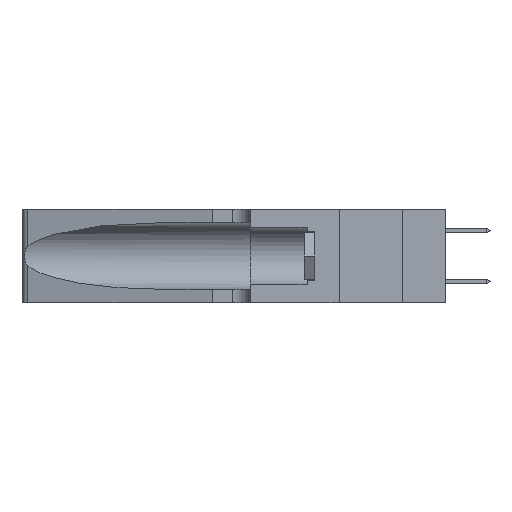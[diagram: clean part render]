
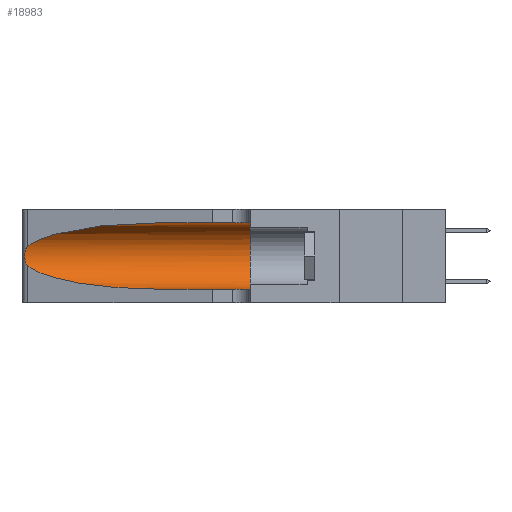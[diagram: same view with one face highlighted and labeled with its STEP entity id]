
A CAD part, left-side view. The second image highlights one B-rep face of the part: STEP entity #18983.
In plain terms, the highlighted cylindrical face has radius 3.308 mm (diameter 6.617 mm), a partial arc.
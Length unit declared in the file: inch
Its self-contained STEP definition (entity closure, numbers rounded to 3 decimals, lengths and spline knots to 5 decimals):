
#10 = FACE_OUTER_BOUND ( 'NONE', #20037, .T. ) ;
#202 = LINE ( 'NONE', #22801, #10548 ) ;
#737 = B_SPLINE_CURVE_WITH_KNOTS ( 'NONE', 3,
 ( #7011, #8962, #22383, #10937, #24310, #12885, #1257, #14824, #3184, #16738, #5118, #18635, #7104, #20547 ),
 .UNSPECIFIED., .F., .F.,
 ( 4, 2, 2, 2, 2, 2, 4 ),
 ( 0., 0.00027, 0.00053, 0.00107, 0.0016, 0.00187, 0.00214 ),
 .UNSPECIFIED. ) ;
#758 = VERTEX_POINT ( 'NONE', #13399 ) ;
#1257 = CARTESIAN_POINT ( 'NONE',  ( 0.26075, 1.23896, 0.19203 ) ) ;
#1822 = AXIS2_PLACEMENT_3D ( 'NONE', #2284, #15841, #4201 ) ;
#2284 = CARTESIAN_POINT ( 'NONE',  ( 0.1305, 0.35, 0.185 ) ) ;
#2355 = CARTESIAN_POINT ( 'NONE',  ( 0.18966, 0.96281, 0.05475 ) ) ;
#3184 = CARTESIAN_POINT ( 'NONE',  ( 0.26017, 1.23833, 0.17102 ) ) ;
#3307 = CARTESIAN_POINT ( 'NONE',  ( 0.1305, 0.72297, 0.31525 ) ) ;
#3493 = DIRECTION ( 'NONE',  ( 0., -1., 0. ) ) ;
#3822 = EDGE_CURVE ( 'NONE', #12488, #758, #737, .T. ) ;
#4157 = CARTESIAN_POINT ( 'NONE',  ( 0.25487, 1.22718, 0.22369 ) ) ;
#4201 = DIRECTION ( 'NONE',  ( 0., 0., 1. ) ) ;
#4568 = CYLINDRICAL_SURFACE ( 'NONE', #11282, 0.13025 ) ;
#5118 = CARTESIAN_POINT ( 'NONE',  ( 0.25789, 1.23486, 0.15765 ) ) ;
#5637 = DIRECTION ( 'NONE',  ( 0., -1., 0. ) ) ;
#5681 =( BOUNDED_CURVE ( )  B_SPLINE_CURVE ( 3, ( #12040, #13962, #2355, #15912 ),
 .UNSPECIFIED., .F., .F. ) 
 B_SPLINE_CURVE_WITH_KNOTS ( ( 4, 4 ),
 ( 3.44316, 4.71239 ),
 .UNSPECIFIED. ) 
 CURVE ( )  GEOMETRIC_REPRESENTATION_ITEM ( )  RATIONAL_B_SPLINE_CURVE ( ( 1., 0.87, 0.87, 1. ) ) 
 REPRESENTATION_ITEM ( '' )  );
#6801 = CARTESIAN_POINT ( 'NONE',  ( 0.1305, 0.72297, 0.05475 ) ) ;
#7011 = CARTESIAN_POINT ( 'NONE',  ( 0.25487, 1.22718, 0.22369 ) ) ;
#7104 = CARTESIAN_POINT ( 'NONE',  ( 0.25555, 1.22993, 0.14849 ) ) ;
#7156 = EDGE_CURVE ( 'NONE', #19584, #22813, #21351, .T. ) ;
#7575 = CARTESIAN_POINT ( 'NONE',  ( 0.1305, 0.35, 0.31525 ) ) ;
#7622 = EDGE_CURVE ( 'NONE', #23781, #19584, #202, .T. ) ;
#7841 = CARTESIAN_POINT ( 'NONE',  ( 0.25487, 1.22718, 0.22369 ) ) ;
#8809 = ORIENTED_EDGE ( 'NONE', *, *, #7622, .F. ) ;
#8962 = CARTESIAN_POINT ( 'NONE',  ( 0.25555, 1.22994, 0.2215 ) ) ;
#10548 = VECTOR ( 'NONE', #18960, 39.37008 ) ;
#10937 = CARTESIAN_POINT ( 'NONE',  ( 0.25787, 1.23484, 0.2124 ) ) ;
#11282 = AXIS2_PLACEMENT_3D ( 'NONE', #22989, #5637, #13385 ) ;
#11324 = ORIENTED_EDGE ( 'NONE', *, *, #7156, .F. ) ;
#11931 = CARTESIAN_POINT ( 'NONE',  ( 0.1305, 0.72297, 0.31525 ) ) ;
#12040 = CARTESIAN_POINT ( 'NONE',  ( 0.25487, 1.22718, 0.14631 ) ) ;
#12488 = VERTEX_POINT ( 'NONE', #7841 ) ;
#12885 = CARTESIAN_POINT ( 'NONE',  ( 0.26018, 1.23835, 0.19895 ) ) ;
#13385 = DIRECTION ( 'NONE',  ( 0., 0., -1. ) ) ;
#13399 = CARTESIAN_POINT ( 'NONE',  ( 0.25487, 1.22718, 0.14631 ) ) ;
#13962 = CARTESIAN_POINT ( 'NONE',  ( 0.2373, 1.15595, 0.08982 ) ) ;
#14727 = ORIENTED_EDGE ( 'NONE', *, *, #19130, .T. ) ;
#14824 = CARTESIAN_POINT ( 'NONE',  ( 0.26075, 1.23896, 0.178 ) ) ;
#14996 = ORIENTED_EDGE ( 'NONE', *, *, #16988, .T. ) ;
#15588 = CARTESIAN_POINT ( 'NONE',  ( 0.1305, 0.35, 0.05475 ) ) ;
#15790 = CARTESIAN_POINT ( 'NONE',  ( 0.2373, 1.15595, 0.28018 ) ) ;
#15841 = DIRECTION ( 'NONE',  ( 0., 1., 0. ) ) ;
#15912 = CARTESIAN_POINT ( 'NONE',  ( 0.1305, 0.72297, 0.05475 ) ) ;
#16291 = ORIENTED_EDGE ( 'NONE', *, *, #3822, .T. ) ;
#16738 = CARTESIAN_POINT ( 'NONE',  ( 0.25856, 1.23593, 0.16098 ) ) ;
#16988 = EDGE_CURVE ( 'NONE', #19942, #22813, #24857, .T. ) ;
#18635 = CARTESIAN_POINT ( 'NONE',  ( 0.25639, 1.23186, 0.15144 ) ) ;
#18940 = CARTESIAN_POINT ( 'NONE',  ( 0.1305, 1.61858, 0.05475 ) ) ;
#18960 = DIRECTION ( 'NONE',  ( 0., -1., 0. ) ) ;
#18983 = ADVANCED_FACE ( 'NONE', ( #10 ), #4568, .F. ) ;
#19130 = EDGE_CURVE ( 'NONE', #758, #19942, #5681, .T. ) ;
#19514 = CARTESIAN_POINT ( 'NONE',  ( 0.18966, 0.96281, 0.31525 ) ) ;
#19584 = VERTEX_POINT ( 'NONE', #7575 ) ;
#19713 = EDGE_CURVE ( 'NONE', #23781, #12488, #21723, .T. ) ;
#19765 = VECTOR ( 'NONE', #3493, 39.37008 ) ;
#19942 = VERTEX_POINT ( 'NONE', #6801 ) ;
#20037 = EDGE_LOOP ( 'NONE', ( #20341, #16291, #14727, #14996, #11324, #8809 ) ) ;
#20341 = ORIENTED_EDGE ( 'NONE', *, *, #19713, .T. ) ;
#20547 = CARTESIAN_POINT ( 'NONE',  ( 0.25487, 1.22718, 0.14631 ) ) ;
#21351 = CIRCLE ( 'NONE', #1822, 0.13025 ) ;
#21723 =( BOUNDED_CURVE ( )  B_SPLINE_CURVE ( 3, ( #11931, #19514, #15790, #4157 ),
 .UNSPECIFIED., .F., .T. ) 
 B_SPLINE_CURVE_WITH_KNOTS ( ( 4, 4 ),
 ( 1.5708, 2.84003 ),
 .UNSPECIFIED. ) 
 CURVE ( )  GEOMETRIC_REPRESENTATION_ITEM ( )  RATIONAL_B_SPLINE_CURVE ( ( 1., 0.87, 0.87, 1. ) ) 
 REPRESENTATION_ITEM ( '' )  );
#22383 = CARTESIAN_POINT ( 'NONE',  ( 0.25639, 1.23184, 0.21858 ) ) ;
#22801 = CARTESIAN_POINT ( 'NONE',  ( 0.1305, 1.61858, 0.31525 ) ) ;
#22813 = VERTEX_POINT ( 'NONE', #15588 ) ;
#22989 = CARTESIAN_POINT ( 'NONE',  ( 0.1305, 1.61858, 0.185 ) ) ;
#23781 = VERTEX_POINT ( 'NONE', #3307 ) ;
#24310 = CARTESIAN_POINT ( 'NONE',  ( 0.25854, 1.2359, 0.20912 ) ) ;
#24857 = LINE ( 'NONE', #18940, #19765 ) ;
